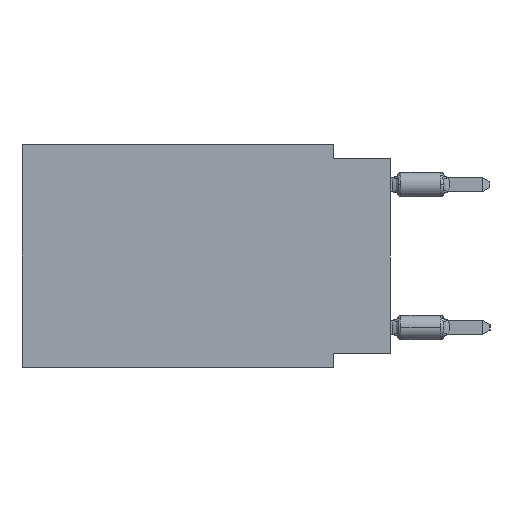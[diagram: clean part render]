
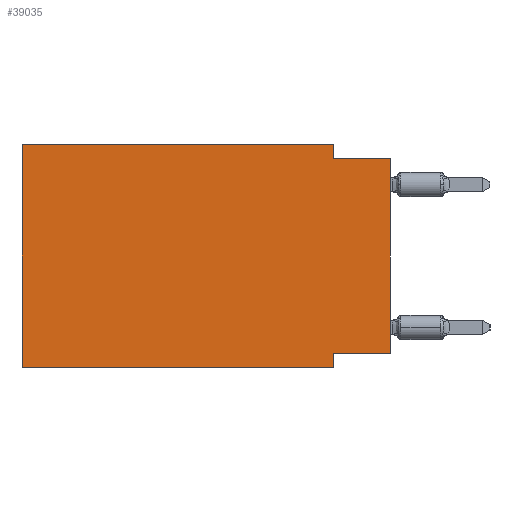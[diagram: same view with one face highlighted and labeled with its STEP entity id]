
A CAD part, left-side view. The second image highlights one B-rep face of the part: STEP entity #39035.
In plain terms, the highlighted planar face has unit normal (-1, 0, 0).
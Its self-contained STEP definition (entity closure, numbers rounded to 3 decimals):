
#105 = ORIENTED_EDGE ( 'NONE', *, *, #48304, .T. ) ;
#762 = LINE ( 'NONE', #46467, #42029 ) ;
#1627 = ORIENTED_EDGE ( 'NONE', *, *, #37701, .T. ) ;
#2563 = VERTEX_POINT ( 'NONE', #20298 ) ;
#2653 = ORIENTED_EDGE ( 'NONE', *, *, #45761, .F. ) ;
#3974 = EDGE_CURVE ( 'NONE', #12140, #48901, #36469, .T. ) ;
#4877 = LINE ( 'NONE', #32110, #28560 ) ;
#4962 = VERTEX_POINT ( 'NONE', #5240 ) ;
#5240 = CARTESIAN_POINT ( 'NONE',  ( 0., 16.383, -9.906 ) ) ;
#5366 = DIRECTION ( 'NONE',  ( 0., -1., 0. ) ) ;
#5909 = CARTESIAN_POINT ( 'NONE',  ( 0., 2.54, -9.271 ) ) ;
#6235 = DIRECTION ( 'NONE',  ( 0., 0., -1. ) ) ;
#6507 = EDGE_CURVE ( 'NONE', #4962, #16971, #41945, .T. ) ;
#6918 = CARTESIAN_POINT ( 'NONE',  ( 0., 16.383, -9.906 ) ) ;
#9721 = LINE ( 'NONE', #24976, #49363 ) ;
#9735 = CARTESIAN_POINT ( 'NONE',  ( 0., 16.383, 0. ) ) ;
#10212 = CARTESIAN_POINT ( 'NONE',  ( 0., 0., -9.271 ) ) ;
#11698 = LINE ( 'NONE', #23708, #32385 ) ;
#12140 = VERTEX_POINT ( 'NONE', #35233 ) ;
#13658 = ORIENTED_EDGE ( 'NONE', *, *, #49325, .F. ) ;
#13736 = VECTOR ( 'NONE', #17698, 1000. ) ;
#14512 = CARTESIAN_POINT ( 'NONE',  ( 0., 0., -0.635 ) ) ;
#15285 = ORIENTED_EDGE ( 'NONE', *, *, #42276, .F. ) ;
#16442 = AXIS2_PLACEMENT_3D ( 'NONE', #9735, #40223, #36986 ) ;
#16971 = VERTEX_POINT ( 'NONE', #20669 ) ;
#17698 = DIRECTION ( 'NONE',  ( 0., 1., 0. ) ) ;
#20298 = CARTESIAN_POINT ( 'NONE',  ( 0., 2.54, -0.635 ) ) ;
#20669 = CARTESIAN_POINT ( 'NONE',  ( 0., 16.383, 0. ) ) ;
#23708 = CARTESIAN_POINT ( 'NONE',  ( 0., 16.383, 0. ) ) ;
#24976 = CARTESIAN_POINT ( 'NONE',  ( 0., 2.54, -9.906 ) ) ;
#25917 = LINE ( 'NONE', #6918, #34684 ) ;
#27039 = EDGE_LOOP ( 'NONE', ( #105, #13658, #46182, #15285, #37111, #1627, #2653, #39249 ) ) ;
#28560 = VECTOR ( 'NONE', #5366, 1000. ) ;
#30239 = DIRECTION ( 'NONE',  ( 0., -1., 0. ) ) ;
#30764 = DIRECTION ( 'NONE',  ( 0., 0., 1. ) ) ;
#31223 = CARTESIAN_POINT ( 'NONE',  ( 0., 16.383, 0. ) ) ;
#32075 = EDGE_CURVE ( 'NONE', #33069, #2563, #39635, .T. ) ;
#32110 = CARTESIAN_POINT ( 'NONE',  ( 0., 0., -0.635 ) ) ;
#32385 = VECTOR ( 'NONE', #30239, 1000. ) ;
#32506 = FACE_OUTER_BOUND ( 'NONE', #27039, .T. ) ;
#32926 = DIRECTION ( 'NONE',  ( 0., -1., 0. ) ) ;
#33069 = VERTEX_POINT ( 'NONE', #40753 ) ;
#34684 = VECTOR ( 'NONE', #32926, 1000. ) ;
#35233 = CARTESIAN_POINT ( 'NONE',  ( 0., 0., -9.271 ) ) ;
#35407 = CARTESIAN_POINT ( 'NONE',  ( 0., 2.54, 0. ) ) ;
#36469 = LINE ( 'NONE', #10212, #13736 ) ;
#36986 = DIRECTION ( 'NONE',  ( 0., 0., -1. ) ) ;
#37111 = ORIENTED_EDGE ( 'NONE', *, *, #6507, .F. ) ;
#37701 = EDGE_CURVE ( 'NONE', #4962, #38820, #25917, .T. ) ;
#38820 = VERTEX_POINT ( 'NONE', #39492 ) ;
#39035 = ADVANCED_FACE ( 'NONE', ( #32506 ), #43972, .F. ) ;
#39249 = ORIENTED_EDGE ( 'NONE', *, *, #3974, .F. ) ;
#39492 = CARTESIAN_POINT ( 'NONE',  ( 0., 2.54, -9.906 ) ) ;
#39631 = VECTOR ( 'NONE', #42937, 1000. ) ;
#39635 = LINE ( 'NONE', #35407, #41206 ) ;
#40223 = DIRECTION ( 'NONE',  ( 1., 0., 0. ) ) ;
#40543 = VERTEX_POINT ( 'NONE', #14512 ) ;
#40753 = CARTESIAN_POINT ( 'NONE',  ( 0., 2.54, 0. ) ) ;
#41206 = VECTOR ( 'NONE', #43620, 1000. ) ;
#41945 = LINE ( 'NONE', #31223, #39631 ) ;
#42029 = VECTOR ( 'NONE', #30764, 1000. ) ;
#42276 = EDGE_CURVE ( 'NONE', #16971, #33069, #11698, .T. ) ;
#42937 = DIRECTION ( 'NONE',  ( 0., 0., 1. ) ) ;
#43620 = DIRECTION ( 'NONE',  ( 0., 0., -1. ) ) ;
#43972 = PLANE ( 'NONE',  #16442 ) ;
#45761 = EDGE_CURVE ( 'NONE', #48901, #38820, #9721, .T. ) ;
#46182 = ORIENTED_EDGE ( 'NONE', *, *, #32075, .F. ) ;
#46467 = CARTESIAN_POINT ( 'NONE',  ( 0., 0., 0. ) ) ;
#48304 = EDGE_CURVE ( 'NONE', #12140, #40543, #762, .T. ) ;
#48901 = VERTEX_POINT ( 'NONE', #5909 ) ;
#49325 = EDGE_CURVE ( 'NONE', #2563, #40543, #4877, .T. ) ;
#49363 = VECTOR ( 'NONE', #6235, 1000. ) ;
